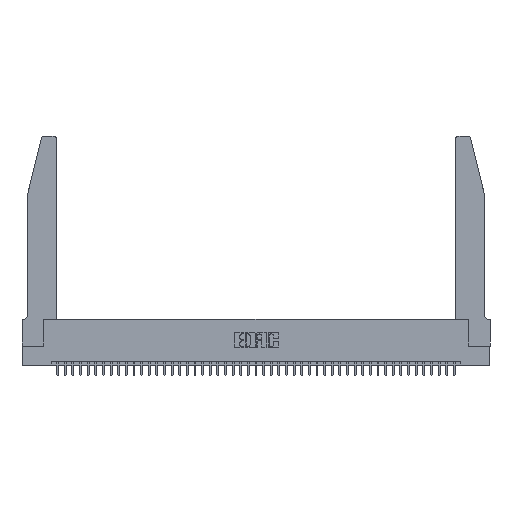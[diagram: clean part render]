
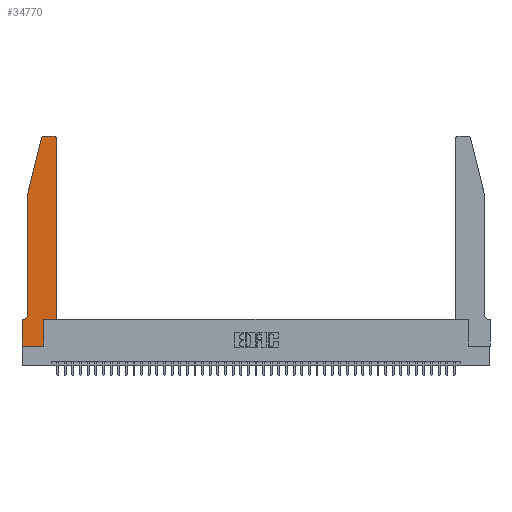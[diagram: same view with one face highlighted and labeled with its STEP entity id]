
A CAD part, top view. The second image highlights one B-rep face of the part: STEP entity #34770.
In plain terms, the highlighted planar face has unit normal (0, 0, 1).
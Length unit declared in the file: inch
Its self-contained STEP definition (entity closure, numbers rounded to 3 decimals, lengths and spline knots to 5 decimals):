
#100 = AXIS2_PLACEMENT_3D ( 'NONE', #2831, #41708, #38779 ) ;
#212 = DIRECTION ( 'NONE',  ( 1., 0., 0. ) ) ;
#1248 = CARTESIAN_POINT ( 'NONE',  ( 0.4205, 2.72, 0.37 ) ) ;
#1430 = DIRECTION ( 'NONE',  ( -1., 0., 0. ) ) ;
#1732 = AXIS2_PLACEMENT_3D ( 'NONE', #1248, #11744, #43328 ) ;
#2147 = EDGE_CURVE ( 'NONE', #40853, #19798, #28359, .T. ) ;
#2589 = ORIENTED_EDGE ( 'NONE', *, *, #30619, .T. ) ;
#2680 = AXIS2_PLACEMENT_3D ( 'NONE', #24469, #11252, #212 ) ;
#2831 = CARTESIAN_POINT ( 'NONE',  ( 0.0055, 0.42, 0.37 ) ) ;
#3845 = LINE ( 'NONE', #24513, #29881 ) ;
#4025 = VECTOR ( 'NONE', #41303, 39.37008 ) ;
#5076 = VECTOR ( 'NONE', #1430, 39.37008 ) ;
#6068 = CARTESIAN_POINT ( 'NONE',  ( 0.0055, 0.35, 0.37 ) ) ;
#6336 = DIRECTION ( 'NONE',  ( 0., 1., 0. ) ) ;
#6352 = CARTESIAN_POINT ( 'NONE',  ( 0.4505, 0.35, 0.37 ) ) ;
#6784 = LINE ( 'NONE', #18564, #19286 ) ;
#6903 = EDGE_CURVE ( 'NONE', #32176, #34671, #26217, .T. ) ;
#7513 = LINE ( 'NONE', #30637, #43426 ) ;
#10928 = CARTESIAN_POINT ( 'NONE',  ( 0.4205, 2.75, 0.37 ) ) ;
#11252 = DIRECTION ( 'NONE',  ( 0., 0., 1. ) ) ;
#11296 = CARTESIAN_POINT ( 'NONE',  ( 0.0755, 0.42, 0.37 ) ) ;
#11638 = EDGE_CURVE ( 'NONE', #21798, #40853, #22423, .T. ) ;
#11744 = DIRECTION ( 'NONE',  ( 0., 0., 1. ) ) ;
#11837 = CARTESIAN_POINT ( 'NONE',  ( 0.4505, 2.72, 0.37 ) ) ;
#12224 = ORIENTED_EDGE ( 'NONE', *, *, #40268, .T. ) ;
#12413 = ORIENTED_EDGE ( 'NONE', *, *, #30098, .T. ) ;
#13638 = PLANE ( 'NONE',  #16791 ) ;
#13751 = EDGE_CURVE ( 'NONE', #16779, #21798, #24943, .T. ) ;
#14441 = ORIENTED_EDGE ( 'NONE', *, *, #13751, .T. ) ;
#14540 = CARTESIAN_POINT ( 'NONE',  ( 0.25487, 2.72718, 0.37 ) ) ;
#16364 = CARTESIAN_POINT ( 'NONE',  ( 0.4505, 0.35, 0.37 ) ) ;
#16779 = VERTEX_POINT ( 'NONE', #11837 ) ;
#16791 = AXIS2_PLACEMENT_3D ( 'NONE', #38229, #38085, #44436 ) ;
#16865 = EDGE_CURVE ( 'NONE', #34671, #39561, #6784, .T. ) ;
#17091 = VERTEX_POINT ( 'NONE', #38471 ) ;
#18564 = CARTESIAN_POINT ( 'NONE',  ( 0.0755, 0.35, 0.37 ) ) ;
#18699 = VERTEX_POINT ( 'NONE', #36954 ) ;
#18980 = VERTEX_POINT ( 'NONE', #39381 ) ;
#19285 = CARTESIAN_POINT ( 'NONE',  ( 0.0755, 2., 0.37 ) ) ;
#19286 = VECTOR ( 'NONE', #36912, 39.37008 ) ;
#19629 = VECTOR ( 'NONE', #44586, 39.37008 ) ;
#19757 = LINE ( 'NONE', #19285, #4025 ) ;
#19781 = VERTEX_POINT ( 'NONE', #39957 ) ;
#19798 = VERTEX_POINT ( 'NONE', #14540 ) ;
#20405 = DIRECTION ( 'NONE',  ( 0., 1., 0. ) ) ;
#20771 = ORIENTED_EDGE ( 'NONE', *, *, #39528, .T. ) ;
#21798 = VERTEX_POINT ( 'NONE', #10928 ) ;
#22423 = LINE ( 'NONE', #29046, #5076 ) ;
#22952 = LINE ( 'NONE', #6352, #19629 ) ;
#22981 = LINE ( 'NONE', #24118, #34866 ) ;
#23762 = CARTESIAN_POINT ( 'NONE',  ( 0., 0.35, 0.37 ) ) ;
#23851 = DIRECTION ( 'NONE',  ( 0., -1., 0. ) ) ;
#24012 = VERTEX_POINT ( 'NONE', #44311 ) ;
#24118 = CARTESIAN_POINT ( 'NONE',  ( 0.0755, 2., 0.37 ) ) ;
#24469 = CARTESIAN_POINT ( 'NONE',  ( 0.284, 2.72, 0.37 ) ) ;
#24510 = ORIENTED_EDGE ( 'NONE', *, *, #2147, .T. ) ;
#24513 = CARTESIAN_POINT ( 'NONE',  ( 0., 0., 0.37 ) ) ;
#24943 = CIRCLE ( 'NONE', #1732, 0.03 ) ;
#24960 = ORIENTED_EDGE ( 'NONE', *, *, #16865, .T. ) ;
#26217 = CIRCLE ( 'NONE', #100, 0.07 ) ;
#26983 = CARTESIAN_POINT ( 'NONE',  ( 0.284, 2.75, 0.37 ) ) ;
#27378 = ORIENTED_EDGE ( 'NONE', *, *, #39054, .T. ) ;
#27870 = DIRECTION ( 'NONE',  ( 1., 0., 0. ) ) ;
#28359 = CIRCLE ( 'NONE', #2680, 0.03 ) ;
#28613 = EDGE_LOOP ( 'NONE', ( #30372, #24510, #2589, #12413, #38107, #24960, #12224, #27378, #29578, #35180, #20771, #14441 ) ) ;
#29046 = CARTESIAN_POINT ( 'NONE',  ( 0.2605, 2.75, 0.37 ) ) ;
#29550 = DIRECTION ( 'NONE',  ( 0., -1., 0. ) ) ;
#29578 = ORIENTED_EDGE ( 'NONE', *, *, #34771, .T. ) ;
#29881 = VECTOR ( 'NONE', #27870, 39.37008 ) ;
#30098 = EDGE_CURVE ( 'NONE', #17091, #32176, #22981, .T. ) ;
#30372 = ORIENTED_EDGE ( 'NONE', *, *, #11638, .T. ) ;
#30619 = EDGE_CURVE ( 'NONE', #19798, #17091, #19757, .T. ) ;
#30637 = CARTESIAN_POINT ( 'NONE',  ( 0., 0., 0.37 ) ) ;
#32176 = VERTEX_POINT ( 'NONE', #11296 ) ;
#34671 = VERTEX_POINT ( 'NONE', #6068 ) ;
#34770 = ADVANCED_FACE ( 'NONE', ( #37879 ), #13638, .T. ) ;
#34771 = EDGE_CURVE ( 'NONE', #18980, #24012, #42211, .T. ) ;
#34866 = VECTOR ( 'NONE', #29550, 39.37008 ) ;
#35180 = ORIENTED_EDGE ( 'NONE', *, *, #36784, .T. ) ;
#35277 = LINE ( 'NONE', #16364, #37512 ) ;
#35630 = VECTOR ( 'NONE', #6336, 39.37008 ) ;
#36784 = EDGE_CURVE ( 'NONE', #24012, #19781, #22952, .T. ) ;
#36912 = DIRECTION ( 'NONE',  ( -1., 0., 0. ) ) ;
#36954 = CARTESIAN_POINT ( 'NONE',  ( 0., 0., 0.37 ) ) ;
#37512 = VECTOR ( 'NONE', #20405, 39.37008 ) ;
#37879 = FACE_OUTER_BOUND ( 'NONE', #28613, .T. ) ;
#37929 = CARTESIAN_POINT ( 'NONE',  ( 0.2865, 0.35, 0.37 ) ) ;
#38085 = DIRECTION ( 'NONE',  ( 0., 0., 1. ) ) ;
#38107 = ORIENTED_EDGE ( 'NONE', *, *, #6903, .T. ) ;
#38229 = CARTESIAN_POINT ( 'NONE',  ( 0., 0.35, 0.37 ) ) ;
#38471 = CARTESIAN_POINT ( 'NONE',  ( 0.0755, 2., 0.37 ) ) ;
#38779 = DIRECTION ( 'NONE',  ( -1., 0., 0. ) ) ;
#39054 = EDGE_CURVE ( 'NONE', #18699, #18980, #3845, .T. ) ;
#39381 = CARTESIAN_POINT ( 'NONE',  ( 0.2865, 0., 0.37 ) ) ;
#39528 = EDGE_CURVE ( 'NONE', #19781, #16779, #35277, .T. ) ;
#39561 = VERTEX_POINT ( 'NONE', #23762 ) ;
#39957 = CARTESIAN_POINT ( 'NONE',  ( 0.4505, 0.35, 0.37 ) ) ;
#40268 = EDGE_CURVE ( 'NONE', #39561, #18699, #7513, .T. ) ;
#40853 = VERTEX_POINT ( 'NONE', #26983 ) ;
#41303 = DIRECTION ( 'NONE',  ( -0.239, -0.971, 0. ) ) ;
#41708 = DIRECTION ( 'NONE',  ( 0., 0., -1. ) ) ;
#42211 = LINE ( 'NONE', #37929, #35630 ) ;
#43328 = DIRECTION ( 'NONE',  ( 1., 0., 0. ) ) ;
#43426 = VECTOR ( 'NONE', #23851, 39.37008 ) ;
#44311 = CARTESIAN_POINT ( 'NONE',  ( 0.2865, 0.35, 0.37 ) ) ;
#44436 = DIRECTION ( 'NONE',  ( 1., 0., 0. ) ) ;
#44586 = DIRECTION ( 'NONE',  ( 1., 0., 0. ) ) ;
